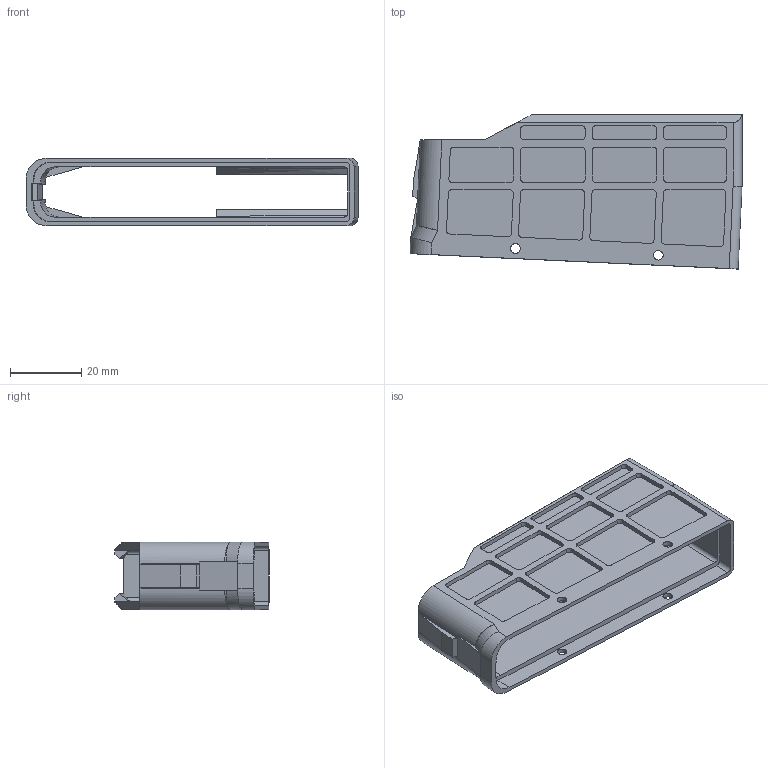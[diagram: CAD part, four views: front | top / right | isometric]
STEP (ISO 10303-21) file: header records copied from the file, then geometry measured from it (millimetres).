
FILE_DESCRIPTION (( 'STEP AP203' ), '1' );
FILE_NAME ('Magazine, Body.STEP', '2013-01-04T08:32:10', ( '' ), ( '' ), 'SwSTEP 2.0', 'SolidWorks 2010', '' );
FILE_SCHEMA (( 'CONFIG_CONTROL_DESIGN' ));
Length unit declared in the file: millimetre
Products named in the file (1): Magazine, Body
Bounding box: 92.89 x 43.1 x 19 mm (x, y, z)
Volume: 13632.9 mm3; surface area: 18664.2 mm2
Topology: 1 solids, 1 shells, 311 faces, 842 edges, 550 vertices
Faces by surface type: plane 173, cylinder 128, bspline 8, sphere 2
Entity records: 10210 total; most frequent: CARTESIAN_POINT 2199, ORIENTED_EDGE 1676, DIRECTION 1644, EDGE_CURVE 838, VECTOR 560, LINE 560, VERTEX_POINT 550, AXIS2_PLACEMENT_3D 542
